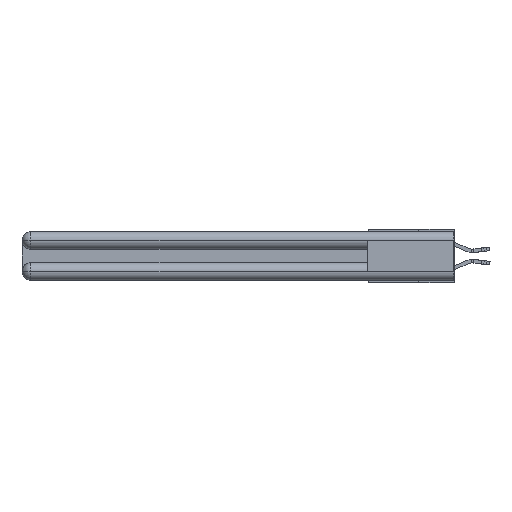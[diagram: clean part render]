
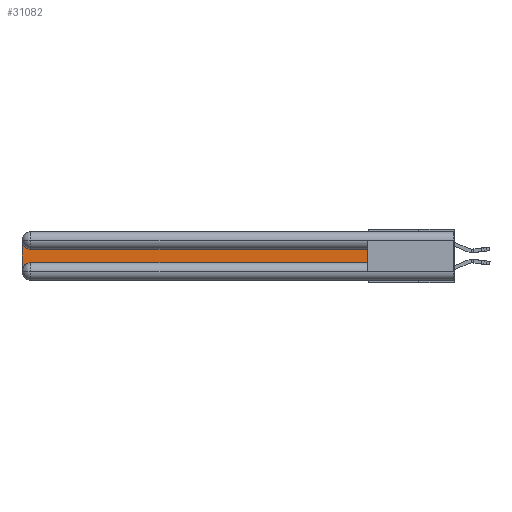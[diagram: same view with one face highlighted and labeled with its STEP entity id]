
A CAD part, left-side view. The second image highlights one B-rep face of the part: STEP entity #31082.
In plain terms, the highlighted planar face has unit normal (-1, 0, 0).
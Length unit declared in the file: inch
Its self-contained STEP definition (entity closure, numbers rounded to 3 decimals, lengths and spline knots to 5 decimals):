
#1192 = DIRECTION ( 'NONE',  ( 0., 0., -1. ) ) ;
#2572 = VERTEX_POINT ( 'NONE', #21602 ) ;
#3185 = VERTEX_POINT ( 'NONE', #8223 ) ;
#5687 = DIRECTION ( 'NONE',  ( 0., 0., -1. ) ) ;
#5776 = DIRECTION ( 'NONE',  ( 0., 1., 0. ) ) ;
#6794 = CARTESIAN_POINT ( 'NONE',  ( 0.075, 0.6, -0.2175 ) ) ;
#7511 = ORIENTED_EDGE ( 'NONE', *, *, #30607, .T. ) ;
#7582 = EDGE_CURVE ( 'NONE', #14704, #2572, #31550, .T. ) ;
#7638 = VECTOR ( 'NONE', #5776, 39.37008 ) ;
#7972 = DIRECTION ( 'NONE',  ( 0., 0., -1. ) ) ;
#8223 = CARTESIAN_POINT ( 'NONE',  ( 0.075, 3., -0.0625 ) ) ;
#8509 = LINE ( 'NONE', #29823, #7638 ) ;
#8757 = DIRECTION ( 'NONE',  ( 1., 0., 0. ) ) ;
#8767 = CARTESIAN_POINT ( 'NONE',  ( 0.075, 0.6, -0.2175 ) ) ;
#9048 = AXIS2_PLACEMENT_3D ( 'NONE', #19357, #8757, #5687 ) ;
#10201 = ORIENTED_EDGE ( 'NONE', *, *, #33744, .T. ) ;
#10541 = EDGE_CURVE ( 'NONE', #28520, #14105, #19692, .T. ) ;
#11699 = EDGE_LOOP ( 'NONE', ( #33696, #22159, #7511, #13334, #10201, #16322 ) ) ;
#13294 = EDGE_CURVE ( 'NONE', #16049, #3185, #28319, .T. ) ;
#13334 = ORIENTED_EDGE ( 'NONE', *, *, #7582, .T. ) ;
#14105 = VERTEX_POINT ( 'NONE', #22022 ) ;
#14202 = VECTOR ( 'NONE', #27996, 39.37008 ) ;
#14566 = VECTOR ( 'NONE', #7972, 39.37008 ) ;
#14704 = VERTEX_POINT ( 'NONE', #29185 ) ;
#16049 = VERTEX_POINT ( 'NONE', #25567 ) ;
#16322 = ORIENTED_EDGE ( 'NONE', *, *, #10541, .T. ) ;
#16563 = EDGE_CURVE ( 'NONE', #14105, #16049, #8509, .T. ) ;
#17152 = VECTOR ( 'NONE', #22563, 39.37008 ) ;
#19357 = CARTESIAN_POINT ( 'NONE',  ( 0.075, 2.94, -0.0625 ) ) ;
#19692 = LINE ( 'NONE', #33783, #14202 ) ;
#20245 = FACE_OUTER_BOUND ( 'NONE', #11699, .T. ) ;
#21602 = CARTESIAN_POINT ( 'NONE',  ( 0.075, 2.94, -0.2175 ) ) ;
#22022 = CARTESIAN_POINT ( 'NONE',  ( 0.075, 0.6, -0.1225 ) ) ;
#22159 = ORIENTED_EDGE ( 'NONE', *, *, #13294, .T. ) ;
#22563 = DIRECTION ( 'NONE',  ( 0., -1., 0. ) ) ;
#24088 = PLANE ( 'NONE',  #29526 ) ;
#24130 = CARTESIAN_POINT ( 'NONE',  ( 0.075, 3., -0.2175 ) ) ;
#25567 = CARTESIAN_POINT ( 'NONE',  ( 0.075, 2.94, -0.1225 ) ) ;
#26543 = AXIS2_PLACEMENT_3D ( 'NONE', #28068, #30777, #1192 ) ;
#27996 = DIRECTION ( 'NONE',  ( 0., 0., 1. ) ) ;
#28068 = CARTESIAN_POINT ( 'NONE',  ( 0.075, 2.94, -0.2775 ) ) ;
#28319 = CIRCLE ( 'NONE', #9048, 0.06 ) ;
#28520 = VERTEX_POINT ( 'NONE', #6794 ) ;
#29185 = CARTESIAN_POINT ( 'NONE',  ( 0.075, 3., -0.2775 ) ) ;
#29526 = AXIS2_PLACEMENT_3D ( 'NONE', #34610, #31865, #32122 ) ;
#29779 = LINE ( 'NONE', #8767, #17152 ) ;
#29823 = CARTESIAN_POINT ( 'NONE',  ( 0.075, 0.6, -0.1225 ) ) ;
#30594 = LINE ( 'NONE', #24130, #14566 ) ;
#30607 = EDGE_CURVE ( 'NONE', #3185, #14704, #30594, .T. ) ;
#30777 = DIRECTION ( 'NONE',  ( 1., 0., 0. ) ) ;
#31082 = ADVANCED_FACE ( 'NONE', ( #20245 ), #24088, .F. ) ;
#31550 = CIRCLE ( 'NONE', #26543, 0.06 ) ;
#31865 = DIRECTION ( 'NONE',  ( 1., 0., 0. ) ) ;
#32122 = DIRECTION ( 'NONE',  ( 0., 0., -1. ) ) ;
#33696 = ORIENTED_EDGE ( 'NONE', *, *, #16563, .T. ) ;
#33744 = EDGE_CURVE ( 'NONE', #2572, #28520, #29779, .T. ) ;
#33783 = CARTESIAN_POINT ( 'NONE',  ( 0.075, 0.6, -0.2175 ) ) ;
#34610 = CARTESIAN_POINT ( 'NONE',  ( 0.075, 3., -0.1225 ) ) ;
